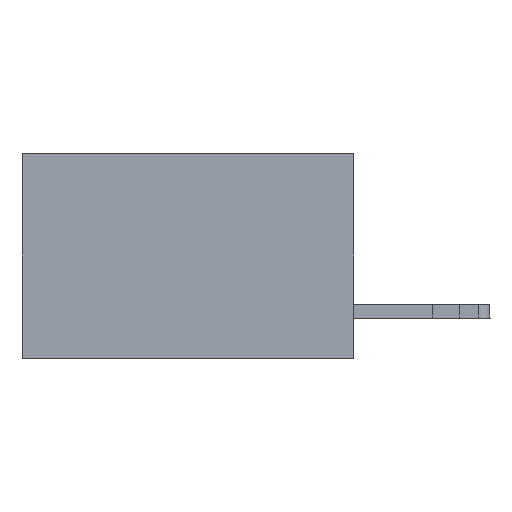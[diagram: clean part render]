
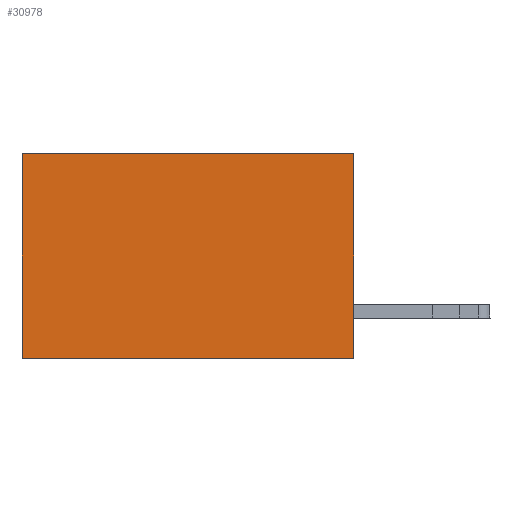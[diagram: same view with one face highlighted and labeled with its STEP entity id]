
A CAD part, left-side view. The second image highlights one B-rep face of the part: STEP entity #30978.
In plain terms, the highlighted planar face has unit normal (-1, 0, 0).
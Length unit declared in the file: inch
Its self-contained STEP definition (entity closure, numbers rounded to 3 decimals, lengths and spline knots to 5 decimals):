
#512 = VERTEX_POINT ( 'NONE', #1237 ) ;
#619 = DIRECTION ( 'NONE',  ( 0., 1., 0. ) ) ;
#1237 = CARTESIAN_POINT ( 'NONE',  ( 0.2875, 0.6, -0.37 ) ) ;
#1250 = LINE ( 'NONE', #20094, #8531 ) ;
#1681 = CARTESIAN_POINT ( 'NONE',  ( 0.2875, 0., -0.37 ) ) ;
#2202 = LINE ( 'NONE', #15119, #8693 ) ;
#2858 = EDGE_LOOP ( 'NONE', ( #3546, #29468, #10430, #13232 ) ) ;
#3422 = CARTESIAN_POINT ( 'NONE',  ( 0.2875, 0.6, 0. ) ) ;
#3546 = ORIENTED_EDGE ( 'NONE', *, *, #27542, .T. ) ;
#6029 = CARTESIAN_POINT ( 'NONE',  ( 0.2875, 0., 0. ) ) ;
#6243 = DIRECTION ( 'NONE',  ( 0., 0., -1. ) ) ;
#6453 = DIRECTION ( 'NONE',  ( 1., 0., 0. ) ) ;
#6479 = AXIS2_PLACEMENT_3D ( 'NONE', #6029, #6453, #6243 ) ;
#8531 = VECTOR ( 'NONE', #15379, 39.37008 ) ;
#8693 = VECTOR ( 'NONE', #619, 39.37008 ) ;
#10430 = ORIENTED_EDGE ( 'NONE', *, *, #31066, .F. ) ;
#13232 = ORIENTED_EDGE ( 'NONE', *, *, #13738, .T. ) ;
#13738 = EDGE_CURVE ( 'NONE', #23374, #26054, #2202, .T. ) ;
#15119 = CARTESIAN_POINT ( 'NONE',  ( 0.2875, 0., 0. ) ) ;
#15379 = DIRECTION ( 'NONE',  ( 0., 1., 0. ) ) ;
#15749 = CARTESIAN_POINT ( 'NONE',  ( 0.2875, 0., 0. ) ) ;
#18736 = LINE ( 'NONE', #20096, #23358 ) ;
#20094 = CARTESIAN_POINT ( 'NONE',  ( 0.2875, 0., -0.37 ) ) ;
#20096 = CARTESIAN_POINT ( 'NONE',  ( 0.2875, 0., 0. ) ) ;
#20596 = EDGE_CURVE ( 'NONE', #21405, #512, #1250, .T. ) ;
#21405 = VERTEX_POINT ( 'NONE', #1681 ) ;
#22472 = DIRECTION ( 'NONE',  ( 0., 0., -1. ) ) ;
#22879 = PLANE ( 'NONE',  #6479 ) ;
#23358 = VECTOR ( 'NONE', #22472, 39.37008 ) ;
#23374 = VERTEX_POINT ( 'NONE', #15749 ) ;
#25185 = VECTOR ( 'NONE', #28137, 39.37008 ) ;
#25259 = CARTESIAN_POINT ( 'NONE',  ( 0.2875, 0.6, 0. ) ) ;
#25981 = LINE ( 'NONE', #3422, #25185 ) ;
#26054 = VERTEX_POINT ( 'NONE', #25259 ) ;
#26464 = FACE_OUTER_BOUND ( 'NONE', #2858, .T. ) ;
#27542 = EDGE_CURVE ( 'NONE', #26054, #512, #25981, .T. ) ;
#28137 = DIRECTION ( 'NONE',  ( 0., 0., -1. ) ) ;
#29468 = ORIENTED_EDGE ( 'NONE', *, *, #20596, .F. ) ;
#30978 = ADVANCED_FACE ( 'NONE', ( #26464 ), #22879, .F. ) ;
#31066 = EDGE_CURVE ( 'NONE', #23374, #21405, #18736, .T. ) ;
